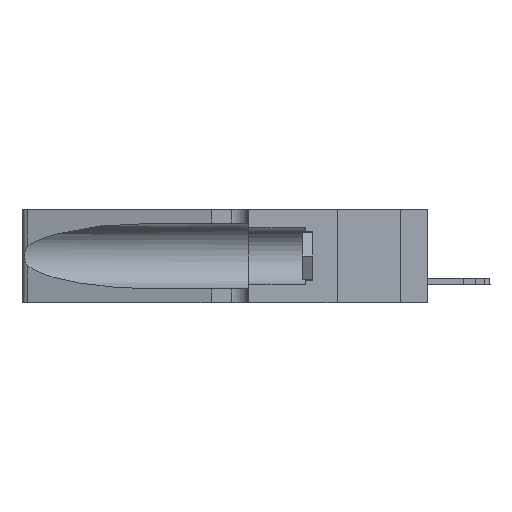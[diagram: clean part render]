
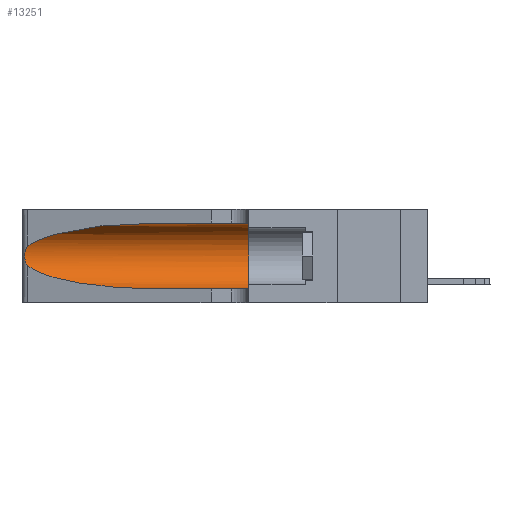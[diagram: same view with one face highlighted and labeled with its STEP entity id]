
A CAD part, left-side view. The second image highlights one B-rep face of the part: STEP entity #13251.
In plain terms, the highlighted cylindrical face has radius 3.308 mm (diameter 6.617 mm), a partial arc.
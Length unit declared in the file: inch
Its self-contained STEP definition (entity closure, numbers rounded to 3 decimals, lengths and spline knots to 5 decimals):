
#230 = VERTEX_POINT ( 'NONE', #12069 ) ;
#374 = DIRECTION ( 'NONE',  ( 0., -1., 0. ) ) ;
#645 = CARTESIAN_POINT ( 'NONE',  ( 0.1305, 0.72297, 0.31525 ) ) ;
#1088 = LINE ( 'NONE', #14972, #13262 ) ;
#1195 = EDGE_CURVE ( 'NONE', #7468, #4140, #21285, .T. ) ;
#1218 = CARTESIAN_POINT ( 'NONE',  ( 0.25487, 1.22718, 0.14631 ) ) ;
#1220 = CARTESIAN_POINT ( 'NONE',  ( 0.25787, 1.23484, 0.2124 ) ) ;
#1482 = AXIS2_PLACEMENT_3D ( 'NONE', #1966, #374, #18817 ) ;
#1643 = CARTESIAN_POINT ( 'NONE',  ( 0.25555, 1.22993, 0.14849 ) ) ;
#1759 = AXIS2_PLACEMENT_3D ( 'NONE', #17219, #19066, #10496 ) ;
#1828 = CARTESIAN_POINT ( 'NONE',  ( 0.1305, 0.72297, 0.31525 ) ) ;
#1966 = CARTESIAN_POINT ( 'NONE',  ( 0.1305, 1.61858, 0.185 ) ) ;
#2094 = EDGE_LOOP ( 'NONE', ( #15110, #13478, #3415, #18495, #19854, #5637 ) ) ;
#2235 = EDGE_CURVE ( 'NONE', #15157, #230, #1088, .T. ) ;
#2677 = CARTESIAN_POINT ( 'NONE',  ( 0.25854, 1.2359, 0.20912 ) ) ;
#3006 = DIRECTION ( 'NONE',  ( 0., -1., 0. ) ) ;
#3236 = CARTESIAN_POINT ( 'NONE',  ( 0.26075, 1.23896, 0.178 ) ) ;
#3415 = ORIENTED_EDGE ( 'NONE', *, *, #17572, .T. ) ;
#4140 = VERTEX_POINT ( 'NONE', #7802 ) ;
#4698 = CARTESIAN_POINT ( 'NONE',  ( 0.1305, 0.35, 0.31525 ) ) ;
#5314 = EDGE_CURVE ( 'NONE', #21070, #7468, #18782, .T. ) ;
#5637 = ORIENTED_EDGE ( 'NONE', *, *, #7417, .F. ) ;
#6784 = CARTESIAN_POINT ( 'NONE',  ( 0.1305, 0.72297, 0.05475 ) ) ;
#6798 = CARTESIAN_POINT ( 'NONE',  ( 0.2373, 1.15595, 0.28018 ) ) ;
#7338 = CYLINDRICAL_SURFACE ( 'NONE', #1482, 0.13025 ) ;
#7417 = EDGE_CURVE ( 'NONE', #21070, #12048, #18180, .T. ) ;
#7468 = VERTEX_POINT ( 'NONE', #17981 ) ;
#7802 = CARTESIAN_POINT ( 'NONE',  ( 0.25487, 1.22718, 0.14631 ) ) ;
#8072 = CARTESIAN_POINT ( 'NONE',  ( 0.25487, 1.22718, 0.14631 ) ) ;
#8429 = CARTESIAN_POINT ( 'NONE',  ( 0.1305, 0.72297, 0.05475 ) ) ;
#10496 = DIRECTION ( 'NONE',  ( 0., 0., 1. ) ) ;
#11528 = CARTESIAN_POINT ( 'NONE',  ( 0.25487, 1.22718, 0.22369 ) ) ;
#11571 = CARTESIAN_POINT ( 'NONE',  ( 0.18966, 0.96281, 0.05475 ) ) ;
#12048 = VERTEX_POINT ( 'NONE', #4698 ) ;
#12069 = CARTESIAN_POINT ( 'NONE',  ( 0.1305, 0.35, 0.05475 ) ) ;
#12615 = CARTESIAN_POINT ( 'NONE',  ( 0.25555, 1.22994, 0.2215 ) ) ;
#12835 = CARTESIAN_POINT ( 'NONE',  ( 0.25639, 1.23184, 0.21858 ) ) ;
#13060 = CIRCLE ( 'NONE', #1759, 0.13025 ) ;
#13214 = CARTESIAN_POINT ( 'NONE',  ( 0.18966, 0.96281, 0.31525 ) ) ;
#13251 = ADVANCED_FACE ( 'NONE', ( #18544 ), #7338, .F. ) ;
#13262 = VECTOR ( 'NONE', #19007, 39.37008 ) ;
#13335 = CARTESIAN_POINT ( 'NONE',  ( 0.1305, 1.61858, 0.31525 ) ) ;
#13478 = ORIENTED_EDGE ( 'NONE', *, *, #1195, .T. ) ;
#13706 = EDGE_CURVE ( 'NONE', #12048, #230, #13060, .T. ) ;
#14211 =( BOUNDED_CURVE ( )  B_SPLINE_CURVE ( 3, ( #1218, #17827, #11571, #8429 ),
 .UNSPECIFIED., .F., .F. ) 
 B_SPLINE_CURVE_WITH_KNOTS ( ( 4, 4 ),
 ( 3.44316, 4.71239 ),
 .UNSPECIFIED. ) 
 CURVE ( )  GEOMETRIC_REPRESENTATION_ITEM ( )  RATIONAL_B_SPLINE_CURVE ( ( 1., 0.87, 0.87, 1. ) ) 
 REPRESENTATION_ITEM ( '' )  );
#14257 = CARTESIAN_POINT ( 'NONE',  ( 0.26075, 1.23896, 0.19203 ) ) ;
#14611 = CARTESIAN_POINT ( 'NONE',  ( 0.25639, 1.23186, 0.15144 ) ) ;
#14685 = CARTESIAN_POINT ( 'NONE',  ( 0.25789, 1.23486, 0.15765 ) ) ;
#14972 = CARTESIAN_POINT ( 'NONE',  ( 0.1305, 1.61858, 0.05475 ) ) ;
#15110 = ORIENTED_EDGE ( 'NONE', *, *, #5314, .T. ) ;
#15157 = VERTEX_POINT ( 'NONE', #6784 ) ;
#16158 = CARTESIAN_POINT ( 'NONE',  ( 0.26018, 1.23835, 0.19895 ) ) ;
#16523 = CARTESIAN_POINT ( 'NONE',  ( 0.26017, 1.23833, 0.17102 ) ) ;
#17219 = CARTESIAN_POINT ( 'NONE',  ( 0.1305, 0.35, 0.185 ) ) ;
#17572 = EDGE_CURVE ( 'NONE', #4140, #15157, #14211, .T. ) ;
#17680 = CARTESIAN_POINT ( 'NONE',  ( 0.25487, 1.22718, 0.22369 ) ) ;
#17827 = CARTESIAN_POINT ( 'NONE',  ( 0.2373, 1.15595, 0.08982 ) ) ;
#17981 = CARTESIAN_POINT ( 'NONE',  ( 0.25487, 1.22718, 0.22369 ) ) ;
#18121 = CARTESIAN_POINT ( 'NONE',  ( 0.25856, 1.23593, 0.16098 ) ) ;
#18180 = LINE ( 'NONE', #13335, #20523 ) ;
#18495 = ORIENTED_EDGE ( 'NONE', *, *, #2235, .T. ) ;
#18544 = FACE_OUTER_BOUND ( 'NONE', #2094, .T. ) ;
#18782 =( BOUNDED_CURVE ( )  B_SPLINE_CURVE ( 3, ( #1828, #13214, #6798, #11528 ),
 .UNSPECIFIED., .F., .F. ) 
 B_SPLINE_CURVE_WITH_KNOTS ( ( 4, 4 ),
 ( 1.5708, 2.84003 ),
 .UNSPECIFIED. ) 
 CURVE ( )  GEOMETRIC_REPRESENTATION_ITEM ( )  RATIONAL_B_SPLINE_CURVE ( ( 1., 0.87, 0.87, 1. ) ) 
 REPRESENTATION_ITEM ( '' )  );
#18817 = DIRECTION ( 'NONE',  ( 0., 0., -1. ) ) ;
#19007 = DIRECTION ( 'NONE',  ( 0., -1., 0. ) ) ;
#19066 = DIRECTION ( 'NONE',  ( 0., 1., 0. ) ) ;
#19854 = ORIENTED_EDGE ( 'NONE', *, *, #13706, .F. ) ;
#20523 = VECTOR ( 'NONE', #3006, 39.37008 ) ;
#21070 = VERTEX_POINT ( 'NONE', #645 ) ;
#21285 = B_SPLINE_CURVE_WITH_KNOTS ( 'NONE', 3,
 ( #17680, #12615, #12835, #1220, #2677, #16158, #14257, #3236, #16523, #18121, #14685, #14611, #1643, #8072 ),
 .UNSPECIFIED., .F., .F.,
 ( 4, 2, 2, 2, 2, 2, 4 ),
 ( 0., 0.00027, 0.00053, 0.00107, 0.0016, 0.00187, 0.00214 ),
 .UNSPECIFIED. ) ;
